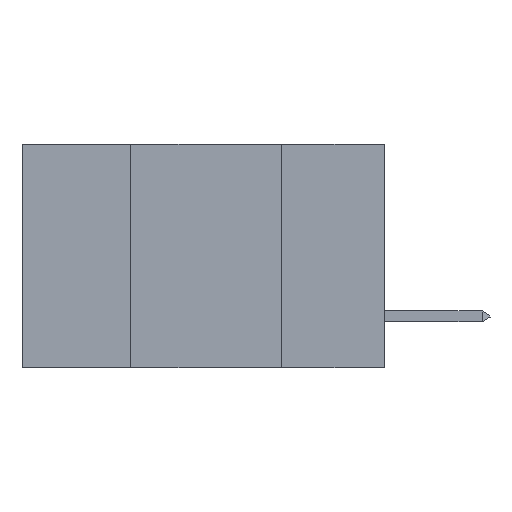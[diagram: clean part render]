
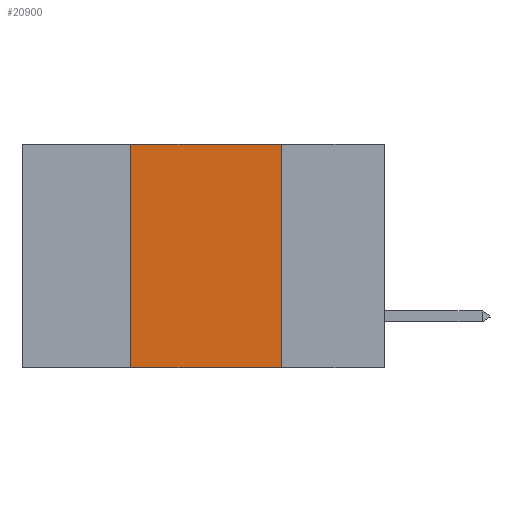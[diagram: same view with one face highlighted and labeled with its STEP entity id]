
A CAD part, left-side view. The second image highlights one B-rep face of the part: STEP entity #20900.
In plain terms, the highlighted planar face has unit normal (-1, 0, 0).
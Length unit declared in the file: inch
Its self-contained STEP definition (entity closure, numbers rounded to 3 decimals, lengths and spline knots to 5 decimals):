
#67 = ORIENTED_EDGE ( 'NONE', *, *, #19928, .F. ) ;
#3167 = LINE ( 'NONE', #12451, #21262 ) ;
#3695 = CARTESIAN_POINT ( 'NONE',  ( 0., 0.17, 0. ) ) ;
#6368 = DIRECTION ( 'NONE',  ( 1., 0., 0. ) ) ;
#6841 = CARTESIAN_POINT ( 'NONE',  ( 0., 0.42, 0. ) ) ;
#7306 = ORIENTED_EDGE ( 'NONE', *, *, #10613, .F. ) ;
#9051 = CARTESIAN_POINT ( 'NONE',  ( 0., 0.42, -0.37 ) ) ;
#9797 = EDGE_CURVE ( 'NONE', #23693, #17885, #25433, .T. ) ;
#10613 = EDGE_CURVE ( 'NONE', #13657, #17885, #18531, .T. ) ;
#10914 = VERTEX_POINT ( 'NONE', #6841 ) ;
#11217 = LINE ( 'NONE', #25679, #14226 ) ;
#12451 = CARTESIAN_POINT ( 'NONE',  ( 0., 0.6, 0. ) ) ;
#12934 = DIRECTION ( 'NONE',  ( 0., -1., 0. ) ) ;
#13657 = VERTEX_POINT ( 'NONE', #3695 ) ;
#14226 = VECTOR ( 'NONE', #17764, 39.37008 ) ;
#16821 = VECTOR ( 'NONE', #20919, 39.37008 ) ;
#17011 = CARTESIAN_POINT ( 'NONE',  ( 0., 0.17, -0.37 ) ) ;
#17274 = CARTESIAN_POINT ( 'NONE',  ( 0., 0.6, 0. ) ) ;
#17360 = ORIENTED_EDGE ( 'NONE', *, *, #18521, .F. ) ;
#17764 = DIRECTION ( 'NONE',  ( 0., 0., 1. ) ) ;
#17885 = VERTEX_POINT ( 'NONE', #17011 ) ;
#18521 = EDGE_CURVE ( 'NONE', #10914, #13657, #3167, .T. ) ;
#18531 = LINE ( 'NONE', #28635, #33058 ) ;
#19919 = DIRECTION ( 'NONE',  ( 0., 0., -1. ) ) ;
#19928 = EDGE_CURVE ( 'NONE', #23693, #10914, #11217, .T. ) ;
#20162 = PLANE ( 'NONE',  #30679 ) ;
#20900 = ADVANCED_FACE ( 'NONE', ( #33442 ), #20162, .F. ) ;
#20919 = DIRECTION ( 'NONE',  ( 0., -1., 0. ) ) ;
#21262 = VECTOR ( 'NONE', #12934, 39.37008 ) ;
#22091 = CARTESIAN_POINT ( 'NONE',  ( 0., 0.6, -0.37 ) ) ;
#23693 = VERTEX_POINT ( 'NONE', #9051 ) ;
#25433 = LINE ( 'NONE', #22091, #16821 ) ;
#25679 = CARTESIAN_POINT ( 'NONE',  ( 0., 0.42, 0. ) ) ;
#26145 = DIRECTION ( 'NONE',  ( 0., 0., -1. ) ) ;
#28635 = CARTESIAN_POINT ( 'NONE',  ( 0., 0.17, 0. ) ) ;
#30679 = AXIS2_PLACEMENT_3D ( 'NONE', #17274, #6368, #19919 ) ;
#33058 = VECTOR ( 'NONE', #26145, 39.37008 ) ;
#33442 = FACE_OUTER_BOUND ( 'NONE', #34077, .T. ) ;
#34077 = EDGE_LOOP ( 'NONE', ( #7306, #17360, #67, #34597 ) ) ;
#34597 = ORIENTED_EDGE ( 'NONE', *, *, #9797, .T. ) ;
